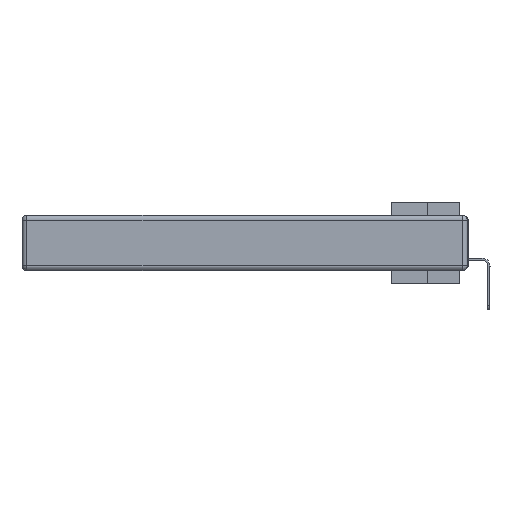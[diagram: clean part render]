
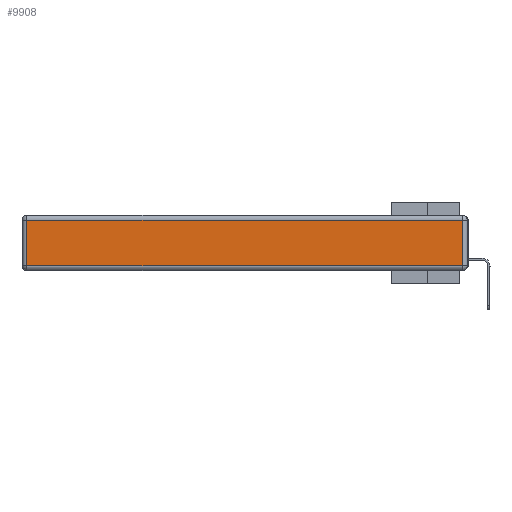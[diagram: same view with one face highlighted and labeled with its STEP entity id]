
A CAD part, left-side view. The second image highlights one B-rep face of the part: STEP entity #9908.
In plain terms, the highlighted planar face has unit normal (-1, 0, 0).
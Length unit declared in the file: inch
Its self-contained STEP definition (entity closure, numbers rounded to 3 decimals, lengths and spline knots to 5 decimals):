
#189 = FACE_OUTER_BOUND ( 'NONE', #34022, .T. ) ;
#233 = CARTESIAN_POINT ( 'NONE',  ( 0., 0.03, -0.03 ) ) ;
#496 = VECTOR ( 'NONE', #24038, 39.37008 ) ;
#1140 = DIRECTION ( 'NONE',  ( 0., 1., 0. ) ) ;
#1386 = CARTESIAN_POINT ( 'NONE',  ( 0., 0., -0.343 ) ) ;
#1562 = VECTOR ( 'NONE', #26701, 39.37008 ) ;
#3106 = LINE ( 'NONE', #19988, #20112 ) ;
#7935 = VERTEX_POINT ( 'NONE', #14161 ) ;
#8431 = CARTESIAN_POINT ( 'NONE',  ( 0., 2.72, -0.03 ) ) ;
#9908 = ADVANCED_FACE ( 'NONE', ( #189 ), #17639, .T. ) ;
#10561 = EDGE_CURVE ( 'NONE', #25878, #17999, #27754, .T. ) ;
#11466 = EDGE_CURVE ( 'NONE', #24464, #25878, #15330, .T. ) ;
#12023 = DIRECTION ( 'NONE',  ( 0., -1., 0. ) ) ;
#13070 = LINE ( 'NONE', #18613, #1562 ) ;
#14161 = CARTESIAN_POINT ( 'NONE',  ( 0., 2.72, -0.313 ) ) ;
#15330 = LINE ( 'NONE', #23919, #496 ) ;
#17432 = DIRECTION ( 'NONE',  ( -1., 0., 0. ) ) ;
#17639 = PLANE ( 'NONE',  #29091 ) ;
#17999 = VERTEX_POINT ( 'NONE', #8431 ) ;
#18167 = ORIENTED_EDGE ( 'NONE', *, *, #22948, .T. ) ;
#18613 = CARTESIAN_POINT ( 'NONE',  ( 0., 2.72, -0.343 ) ) ;
#19988 = CARTESIAN_POINT ( 'NONE',  ( 0., 0., -0.313 ) ) ;
#20112 = VECTOR ( 'NONE', #12023, 39.37008 ) ;
#20490 = VECTOR ( 'NONE', #1140, 39.37008 ) ;
#22948 = EDGE_CURVE ( 'NONE', #7935, #24464, #3106, .T. ) ;
#23083 = CARTESIAN_POINT ( 'NONE',  ( 0., 2.75, -0.03 ) ) ;
#23257 = ORIENTED_EDGE ( 'NONE', *, *, #11466, .T. ) ;
#23919 = CARTESIAN_POINT ( 'NONE',  ( 0., 0.03, -0.343 ) ) ;
#24038 = DIRECTION ( 'NONE',  ( 0., 0., 1. ) ) ;
#24144 = CARTESIAN_POINT ( 'NONE',  ( 0., 0.03, -0.313 ) ) ;
#24464 = VERTEX_POINT ( 'NONE', #24144 ) ;
#25878 = VERTEX_POINT ( 'NONE', #233 ) ;
#26701 = DIRECTION ( 'NONE',  ( 0., 0., -1. ) ) ;
#27754 = LINE ( 'NONE', #23083, #20490 ) ;
#29091 = AXIS2_PLACEMENT_3D ( 'NONE', #1386, #17432, #33487 ) ;
#30769 = ORIENTED_EDGE ( 'NONE', *, *, #10561, .T. ) ;
#32265 = EDGE_CURVE ( 'NONE', #17999, #7935, #13070, .T. ) ;
#33487 = DIRECTION ( 'NONE',  ( 0., 0., 1. ) ) ;
#33880 = ORIENTED_EDGE ( 'NONE', *, *, #32265, .T. ) ;
#34022 = EDGE_LOOP ( 'NONE', ( #18167, #23257, #30769, #33880 ) ) ;
